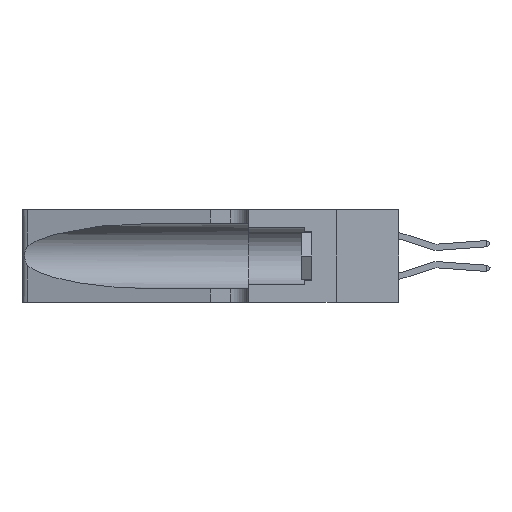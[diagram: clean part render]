
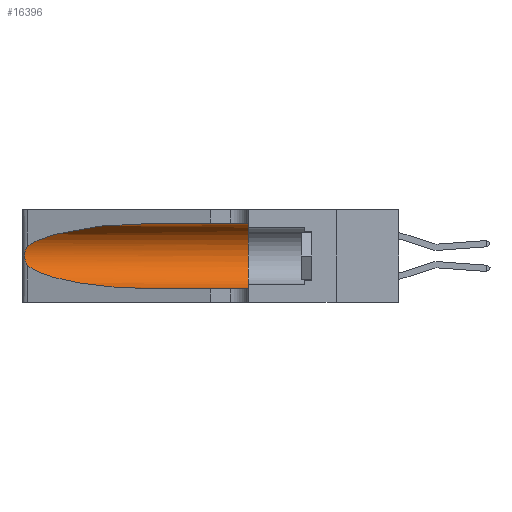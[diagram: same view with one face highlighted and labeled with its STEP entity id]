
A CAD part, left-side view. The second image highlights one B-rep face of the part: STEP entity #16396.
In plain terms, the highlighted cylindrical face has radius 3.308 mm (diameter 6.617 mm), a partial arc.
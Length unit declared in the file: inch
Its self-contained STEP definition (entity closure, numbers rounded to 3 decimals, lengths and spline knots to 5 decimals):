
#283 = CARTESIAN_POINT ( 'NONE',  ( 0.1305, 0.72297, 0.05475 ) ) ;
#295 =( BOUNDED_CURVE ( )  B_SPLINE_CURVE ( 3, ( #17089, #11698, #9318, #21899 ),
 .UNSPECIFIED., .F., .T. ) 
 B_SPLINE_CURVE_WITH_KNOTS ( ( 4, 4 ),
 ( 1.5708, 2.84003 ),
 .UNSPECIFIED. ) 
 CURVE ( )  GEOMETRIC_REPRESENTATION_ITEM ( )  RATIONAL_B_SPLINE_CURVE ( ( 1., 0.87, 0.87, 1. ) ) 
 REPRESENTATION_ITEM ( '' )  );
#375 = CARTESIAN_POINT ( 'NONE',  ( 0.25487, 1.22718, 0.14631 ) ) ;
#537 = AXIS2_PLACEMENT_3D ( 'NONE', #14541, #17119, #1671 ) ;
#724 = LINE ( 'NONE', #7021, #18529 ) ;
#728 = EDGE_CURVE ( 'NONE', #14527, #28444, #4207, .T. ) ;
#1350 = ORIENTED_EDGE ( 'NONE', *, *, #15988, .F. ) ;
#1671 = DIRECTION ( 'NONE',  ( 0., 0., 1. ) ) ;
#1988 = CARTESIAN_POINT ( 'NONE',  ( 0.1305, 1.61858, 0.185 ) ) ;
#3796 = VECTOR ( 'NONE', #7953, 39.37008 ) ;
#4207 =( BOUNDED_CURVE ( )  B_SPLINE_CURVE ( 3, ( #375, #23668, #8250, #283 ),
 .UNSPECIFIED., .F., .T. ) 
 B_SPLINE_CURVE_WITH_KNOTS ( ( 4, 4 ),
 ( 3.44316, 4.71239 ),
 .UNSPECIFIED. ) 
 CURVE ( )  GEOMETRIC_REPRESENTATION_ITEM ( )  RATIONAL_B_SPLINE_CURVE ( ( 1., 0.87, 0.87, 1. ) ) 
 REPRESENTATION_ITEM ( '' )  );
#5683 = EDGE_CURVE ( 'NONE', #28444, #24590, #724, .T. ) ;
#5918 = AXIS2_PLACEMENT_3D ( 'NONE', #1988, #24151, #26821 ) ;
#7021 = CARTESIAN_POINT ( 'NONE',  ( 0.1305, 1.61858, 0.05475 ) ) ;
#7500 = VERTEX_POINT ( 'NONE', #9884 ) ;
#7850 = CARTESIAN_POINT ( 'NONE',  ( 0.1305, 1.61858, 0.31525 ) ) ;
#7953 = DIRECTION ( 'NONE',  ( 0., -1., 0. ) ) ;
#8250 = CARTESIAN_POINT ( 'NONE',  ( 0.18966, 0.96281, 0.05475 ) ) ;
#8501 = CARTESIAN_POINT ( 'NONE',  ( 0.25787, 1.23484, 0.2124 ) ) ;
#8602 = CARTESIAN_POINT ( 'NONE',  ( 0.25487, 1.22718, 0.22369 ) ) ;
#9147 = CARTESIAN_POINT ( 'NONE',  ( 0.25487, 1.22718, 0.22369 ) ) ;
#9318 = CARTESIAN_POINT ( 'NONE',  ( 0.2373, 1.15595, 0.28018 ) ) ;
#9510 = LINE ( 'NONE', #7850, #3796 ) ;
#9884 = CARTESIAN_POINT ( 'NONE',  ( 0.1305, 0.35, 0.31525 ) ) ;
#9942 = EDGE_CURVE ( 'NONE', #22772, #12278, #295, .T. ) ;
#10689 = CARTESIAN_POINT ( 'NONE',  ( 0.25487, 1.22718, 0.14631 ) ) ;
#11021 = ORIENTED_EDGE ( 'NONE', *, *, #23059, .F. ) ;
#11095 = CARTESIAN_POINT ( 'NONE',  ( 0.25789, 1.23486, 0.15765 ) ) ;
#11151 = EDGE_LOOP ( 'NONE', ( #27798, #30828, #18178, #21505, #11021, #1350 ) ) ;
#11279 = CARTESIAN_POINT ( 'NONE',  ( 0.1305, 0.72297, 0.05475 ) ) ;
#11698 = CARTESIAN_POINT ( 'NONE',  ( 0.18966, 0.96281, 0.31525 ) ) ;
#12278 = VERTEX_POINT ( 'NONE', #9147 ) ;
#14527 = VERTEX_POINT ( 'NONE', #10689 ) ;
#14541 = CARTESIAN_POINT ( 'NONE',  ( 0.1305, 0.35, 0.185 ) ) ;
#15160 = EDGE_CURVE ( 'NONE', #12278, #14527, #26638, .T. ) ;
#15689 = CARTESIAN_POINT ( 'NONE',  ( 0.1305, 0.35, 0.05475 ) ) ;
#15988 = EDGE_CURVE ( 'NONE', #22772, #7500, #9510, .T. ) ;
#16392 = CARTESIAN_POINT ( 'NONE',  ( 0.25555, 1.22993, 0.14849 ) ) ;
#16396 = ADVANCED_FACE ( 'NONE', ( #19503 ), #21097, .F. ) ;
#17089 = CARTESIAN_POINT ( 'NONE',  ( 0.1305, 0.72297, 0.31525 ) ) ;
#17119 = DIRECTION ( 'NONE',  ( 0., 1., 0. ) ) ;
#18178 = ORIENTED_EDGE ( 'NONE', *, *, #728, .T. ) ;
#18529 = VECTOR ( 'NONE', #26099, 39.37008 ) ;
#18542 = CARTESIAN_POINT ( 'NONE',  ( 0.25555, 1.22994, 0.2215 ) ) ;
#18644 = CARTESIAN_POINT ( 'NONE',  ( 0.25854, 1.2359, 0.20912 ) ) ;
#18863 = CARTESIAN_POINT ( 'NONE',  ( 0.26018, 1.23835, 0.19895 ) ) ;
#19503 = FACE_OUTER_BOUND ( 'NONE', #11151, .T. ) ;
#21097 = CYLINDRICAL_SURFACE ( 'NONE', #5918, 0.13025 ) ;
#21122 = CARTESIAN_POINT ( 'NONE',  ( 0.26075, 1.23896, 0.19203 ) ) ;
#21505 = ORIENTED_EDGE ( 'NONE', *, *, #5683, .T. ) ;
#21557 = CARTESIAN_POINT ( 'NONE',  ( 0.26075, 1.23896, 0.178 ) ) ;
#21899 = CARTESIAN_POINT ( 'NONE',  ( 0.25487, 1.22718, 0.22369 ) ) ;
#22772 = VERTEX_POINT ( 'NONE', #32954 ) ;
#23059 = EDGE_CURVE ( 'NONE', #7500, #24590, #28540, .T. ) ;
#23668 = CARTESIAN_POINT ( 'NONE',  ( 0.2373, 1.15595, 0.08982 ) ) ;
#24151 = DIRECTION ( 'NONE',  ( 0., -1., 0. ) ) ;
#24590 = VERTEX_POINT ( 'NONE', #15689 ) ;
#26099 = DIRECTION ( 'NONE',  ( 0., -1., 0. ) ) ;
#26460 = CARTESIAN_POINT ( 'NONE',  ( 0.26017, 1.23833, 0.17102 ) ) ;
#26638 = B_SPLINE_CURVE_WITH_KNOTS ( 'NONE', 3,
 ( #8602, #18542, #31734, #8501, #18644, #18863, #21122, #21557, #26460, #28906, #11095, #29011, #16392, #31303 ),
 .UNSPECIFIED., .F., .F.,
 ( 4, 2, 2, 2, 2, 2, 4 ),
 ( 0., 0.00027, 0.00053, 0.00107, 0.0016, 0.00187, 0.00214 ),
 .UNSPECIFIED. ) ;
#26821 = DIRECTION ( 'NONE',  ( 0., 0., -1. ) ) ;
#27798 = ORIENTED_EDGE ( 'NONE', *, *, #9942, .T. ) ;
#28444 = VERTEX_POINT ( 'NONE', #11279 ) ;
#28540 = CIRCLE ( 'NONE', #537, 0.13025 ) ;
#28906 = CARTESIAN_POINT ( 'NONE',  ( 0.25856, 1.23593, 0.16098 ) ) ;
#29011 = CARTESIAN_POINT ( 'NONE',  ( 0.25639, 1.23186, 0.15144 ) ) ;
#30828 = ORIENTED_EDGE ( 'NONE', *, *, #15160, .T. ) ;
#31303 = CARTESIAN_POINT ( 'NONE',  ( 0.25487, 1.22718, 0.14631 ) ) ;
#31734 = CARTESIAN_POINT ( 'NONE',  ( 0.25639, 1.23184, 0.21858 ) ) ;
#32954 = CARTESIAN_POINT ( 'NONE',  ( 0.1305, 0.72297, 0.31525 ) ) ;
